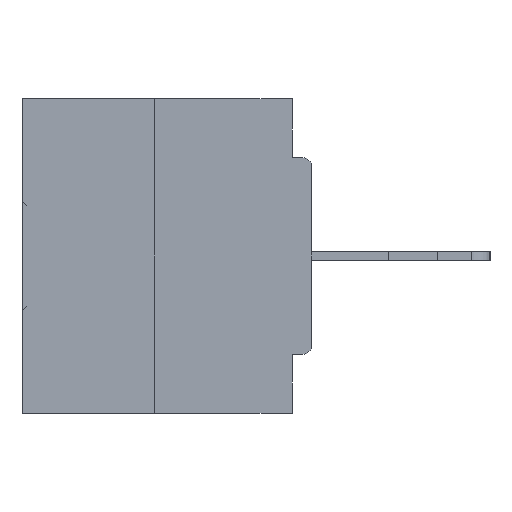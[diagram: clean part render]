
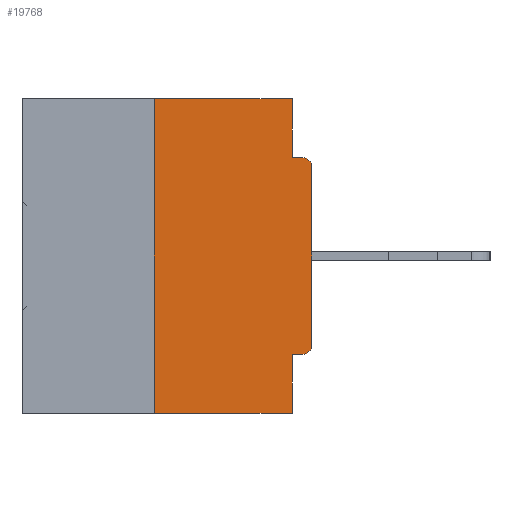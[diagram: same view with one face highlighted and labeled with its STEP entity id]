
A CAD part, left-side view. The second image highlights one B-rep face of the part: STEP entity #19768.
In plain terms, the highlighted planar face has unit normal (-1, 0, 0).
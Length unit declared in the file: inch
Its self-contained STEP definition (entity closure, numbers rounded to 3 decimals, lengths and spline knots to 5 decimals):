
#288 = VECTOR ( 'NONE', #7095, 39.37008 ) ;
#992 = DIRECTION ( 'NONE',  ( 0., -1., 0. ) ) ;
#1214 = DIRECTION ( 'NONE',  ( 0., 0., 1. ) ) ;
#1468 = LINE ( 'NONE', #17755, #31803 ) ;
#2046 = CARTESIAN_POINT ( 'NONE',  ( 0., 0., 0. ) ) ;
#2917 = AXIS2_PLACEMENT_3D ( 'NONE', #31737, #6052, #3110 ) ;
#3110 = DIRECTION ( 'NONE',  ( 0., 0., -1. ) ) ;
#3549 = EDGE_CURVE ( 'NONE', #8936, #39898, #15876, .T. ) ;
#3596 = CARTESIAN_POINT ( 'NONE',  ( 0., 0., -0.3915 ) ) ;
#3915 = CARTESIAN_POINT ( 'NONE',  ( 0., 0., -0.0935 ) ) ;
#4272 = CARTESIAN_POINT ( 'NONE',  ( 0., 0.015, -0.0935 ) ) ;
#4318 = DIRECTION ( 'NONE',  ( 0., 0., -1. ) ) ;
#4625 = LINE ( 'NONE', #27189, #17718 ) ;
#4875 = EDGE_CURVE ( 'NONE', #35174, #8936, #10241, .T. ) ;
#6052 = DIRECTION ( 'NONE',  ( -1., 0., 0. ) ) ;
#6352 = VERTEX_POINT ( 'NONE', #20518 ) ;
#6588 = EDGE_CURVE ( 'NONE', #39898, #19525, #39644, .T. ) ;
#7095 = DIRECTION ( 'NONE',  ( 0., -1., 0. ) ) ;
#7620 = DIRECTION ( 'NONE',  ( 0., 0., -1. ) ) ;
#8836 = ORIENTED_EDGE ( 'NONE', *, *, #31044, .F. ) ;
#8936 = VERTEX_POINT ( 'NONE', #21669 ) ;
#9029 = ORIENTED_EDGE ( 'NONE', *, *, #3549, .F. ) ;
#9179 = ORIENTED_EDGE ( 'NONE', *, *, #31423, .F. ) ;
#9720 = CARTESIAN_POINT ( 'NONE',  ( 0., 0.25, -0.5 ) ) ;
#9979 = VECTOR ( 'NONE', #992, 39.37008 ) ;
#10241 = LINE ( 'NONE', #35710, #288 ) ;
#10817 = VERTEX_POINT ( 'NONE', #33682 ) ;
#11465 = VERTEX_POINT ( 'NONE', #20610 ) ;
#11593 = FACE_OUTER_BOUND ( 'NONE', #20780, .T. ) ;
#11727 = VERTEX_POINT ( 'NONE', #9720 ) ;
#11867 = CARTESIAN_POINT ( 'NONE',  ( 0., 0., -0.4065 ) ) ;
#12919 = ORIENTED_EDGE ( 'NONE', *, *, #19165, .T. ) ;
#13554 = LINE ( 'NONE', #35271, #15386 ) ;
#13650 = ORIENTED_EDGE ( 'NONE', *, *, #17614, .T. ) ;
#13731 = DIRECTION ( 'NONE',  ( -1., 0., 0. ) ) ;
#14368 = AXIS2_PLACEMENT_3D ( 'NONE', #29612, #13731, #4318 ) ;
#14993 = ORIENTED_EDGE ( 'NONE', *, *, #21850, .F. ) ;
#15386 = VECTOR ( 'NONE', #1214, 39.37008 ) ;
#15507 = CARTESIAN_POINT ( 'NONE',  ( 0., 0.031, -0.4065 ) ) ;
#15876 = LINE ( 'NONE', #35080, #38719 ) ;
#16992 = AXIS2_PLACEMENT_3D ( 'NONE', #23510, #36239, #7620 ) ;
#17364 = EDGE_CURVE ( 'NONE', #6352, #19525, #22932, .T. ) ;
#17614 = EDGE_CURVE ( 'NONE', #34995, #6352, #30665, .T. ) ;
#17718 = VECTOR ( 'NONE', #39943, 39.37008 ) ;
#17755 = CARTESIAN_POINT ( 'NONE',  ( 0., 0.031, -0.5 ) ) ;
#18402 = ORIENTED_EDGE ( 'NONE', *, *, #6588, .F. ) ;
#19165 = EDGE_CURVE ( 'NONE', #11465, #34995, #28375, .T. ) ;
#19525 = VERTEX_POINT ( 'NONE', #4272 ) ;
#19768 = ADVANCED_FACE ( 'NONE', ( #11593 ), #26623, .F. ) ;
#20518 = CARTESIAN_POINT ( 'NONE',  ( 0., 0., -0.1085 ) ) ;
#20610 = CARTESIAN_POINT ( 'NONE',  ( 0., 0.015, -0.4065 ) ) ;
#20780 = EDGE_LOOP ( 'NONE', ( #33944, #8836, #34223, #14993, #9179, #12919, #13650, #37366, #18402, #9029 ) ) ;
#21669 = CARTESIAN_POINT ( 'NONE',  ( 0., 0.031, 0. ) ) ;
#21850 = EDGE_CURVE ( 'NONE', #26178, #10817, #1468, .T. ) ;
#22932 = CIRCLE ( 'NONE', #2917, 0.015 ) ;
#22961 = VECTOR ( 'NONE', #28306, 39.37008 ) ;
#23124 = EDGE_CURVE ( 'NONE', #11727, #10817, #4625, .T. ) ;
#23510 = CARTESIAN_POINT ( 'NONE',  ( 0., 0.46, 0. ) ) ;
#23651 = CARTESIAN_POINT ( 'NONE',  ( 0., 0.25, 0. ) ) ;
#23819 = DIRECTION ( 'NONE',  ( 0., 0., -1. ) ) ;
#24602 = DIRECTION ( 'NONE',  ( 0., 1., 0. ) ) ;
#26178 = VERTEX_POINT ( 'NONE', #15507 ) ;
#26623 = PLANE ( 'NONE',  #16992 ) ;
#27189 = CARTESIAN_POINT ( 'NONE',  ( 0., 0.46, -0.5 ) ) ;
#28306 = DIRECTION ( 'NONE',  ( 0., 0., 1. ) ) ;
#28375 = CIRCLE ( 'NONE', #14368, 0.015 ) ;
#29612 = CARTESIAN_POINT ( 'NONE',  ( 0., 0.015, -0.3915 ) ) ;
#30665 = LINE ( 'NONE', #2046, #22961 ) ;
#31044 = EDGE_CURVE ( 'NONE', #11727, #35174, #13554, .T. ) ;
#31418 = CARTESIAN_POINT ( 'NONE',  ( 0., 0.031, -0.0935 ) ) ;
#31423 = EDGE_CURVE ( 'NONE', #11465, #26178, #40491, .T. ) ;
#31737 = CARTESIAN_POINT ( 'NONE',  ( 0., 0.015, -0.1085 ) ) ;
#31803 = VECTOR ( 'NONE', #23819, 39.37008 ) ;
#33682 = CARTESIAN_POINT ( 'NONE',  ( 0., 0.031, -0.5 ) ) ;
#33944 = ORIENTED_EDGE ( 'NONE', *, *, #4875, .F. ) ;
#34223 = ORIENTED_EDGE ( 'NONE', *, *, #23124, .T. ) ;
#34679 = DIRECTION ( 'NONE',  ( 0., 0., -1. ) ) ;
#34995 = VERTEX_POINT ( 'NONE', #3596 ) ;
#35080 = CARTESIAN_POINT ( 'NONE',  ( 0., 0.031, 0. ) ) ;
#35174 = VERTEX_POINT ( 'NONE', #23651 ) ;
#35271 = CARTESIAN_POINT ( 'NONE',  ( 0., 0.25, 0. ) ) ;
#35710 = CARTESIAN_POINT ( 'NONE',  ( 0., 0.46, 0. ) ) ;
#36068 = VECTOR ( 'NONE', #24602, 39.37008 ) ;
#36239 = DIRECTION ( 'NONE',  ( 1., 0., 0. ) ) ;
#37366 = ORIENTED_EDGE ( 'NONE', *, *, #17364, .T. ) ;
#38719 = VECTOR ( 'NONE', #34679, 39.37008 ) ;
#39644 = LINE ( 'NONE', #3915, #9979 ) ;
#39898 = VERTEX_POINT ( 'NONE', #31418 ) ;
#39943 = DIRECTION ( 'NONE',  ( 0., -1., 0. ) ) ;
#40491 = LINE ( 'NONE', #11867, #36068 ) ;
